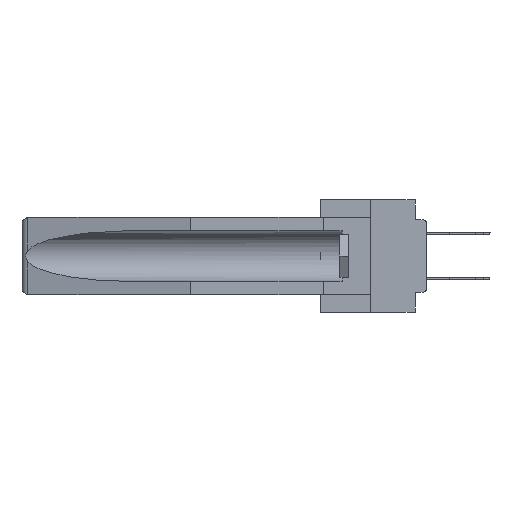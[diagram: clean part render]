
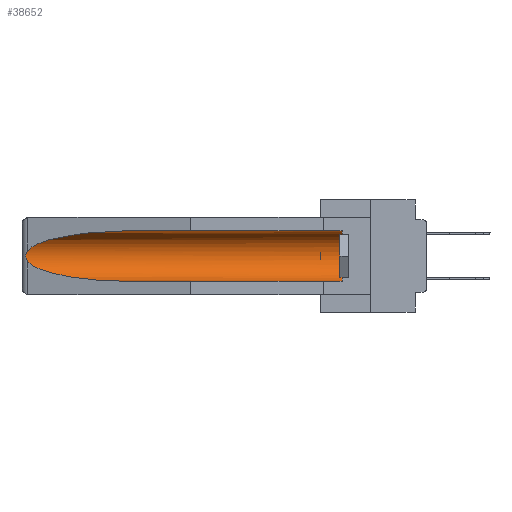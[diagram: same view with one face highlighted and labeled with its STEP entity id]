
A CAD part, left-side view. The second image highlights one B-rep face of the part: STEP entity #38652.
In plain terms, the highlighted cylindrical face has radius 2.857 mm (diameter 5.715 mm), a partial arc.
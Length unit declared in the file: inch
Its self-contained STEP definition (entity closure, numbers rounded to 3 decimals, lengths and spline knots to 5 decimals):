
#609 = CARTESIAN_POINT ( 'NONE',  ( 0.26654, 1.53092, -0.15636 ) ) ;
#806 = CARTESIAN_POINT ( 'NONE',  ( 0.26655, 1.53094, -0.18657 ) ) ;
#1081 = CARTESIAN_POINT ( 'NONE',  ( 0.26537, 1.52718, -0.14972 ) ) ;
#1139 = CARTESIAN_POINT ( 'NONE',  ( 0.155, -0.30754, -0.284 ) ) ;
#1728 = ORIENTED_EDGE ( 'NONE', *, *, #10005, .T. ) ;
#3050 = AXIS2_PLACEMENT_3D ( 'NONE', #12891, #9773, #9546 ) ;
#3756 = CARTESIAN_POINT ( 'NONE',  ( 0.26537, 1.52718, -0.14972 ) ) ;
#4275 = DIRECTION ( 'NONE',  ( 0., 1., 0. ) ) ;
#4434 = CARTESIAN_POINT ( 'NONE',  ( 0.155, 1.07973, -0.059 ) ) ;
#4891 = CARTESIAN_POINT ( 'NONE',  ( 0.155, -0.30754, -0.1715 ) ) ;
#5261 = CARTESIAN_POINT ( 'NONE',  ( 0.21114, 1.30732, -0.284 ) ) ;
#5456 = CARTESIAN_POINT ( 'NONE',  ( 0.26537, 1.52718, -0.19328 ) ) ;
#5550 = EDGE_CURVE ( 'NONE', #35433, #32252, #39615, .T. ) ;
#5663 = CARTESIAN_POINT ( 'NONE',  ( 0.155, 0.126, -0.284 ) ) ;
#6331 = EDGE_CURVE ( 'NONE', #32613, #35433, #33006, .T. ) ;
#7255 = VECTOR ( 'NONE', #4275, 39.37008 ) ;
#7978 = CARTESIAN_POINT ( 'NONE',  ( 0.155, 1.07973, -0.284 ) ) ;
#8008 = CARTESIAN_POINT ( 'NONE',  ( 0.155, 1.07973, -0.059 ) ) ;
#8222 = FACE_OUTER_BOUND ( 'NONE', #16572, .T. ) ;
#8805 = ORIENTED_EDGE ( 'NONE', *, *, #15074, .T. ) ;
#9546 = DIRECTION ( 'NONE',  ( 0., 0., 1. ) ) ;
#9773 = DIRECTION ( 'NONE',  ( 0., -1., 0. ) ) ;
#9837 = AXIS2_PLACEMENT_3D ( 'NONE', #4891, #21392, #27253 ) ;
#10005 = EDGE_CURVE ( 'NONE', #35949, #32613, #24362, .T. ) ;
#12891 = CARTESIAN_POINT ( 'NONE',  ( 0.155, 0.126, -0.1715 ) ) ;
#13347 = CARTESIAN_POINT ( 'NONE',  ( 0.2675, 1.53308, -0.17534 ) ) ;
#13971 = CARTESIAN_POINT ( 'NONE',  ( 0.155, 1.07973, -0.284 ) ) ;
#14422 = ORIENTED_EDGE ( 'NONE', *, *, #19055, .T. ) ;
#14538 = CARTESIAN_POINT ( 'NONE',  ( 0.2673, 1.53269, -0.17917 ) ) ;
#15074 = EDGE_CURVE ( 'NONE', #34534, #35949, #24434, .T. ) ;
#16488 = CARTESIAN_POINT ( 'NONE',  ( 0.26537, 1.52718, -0.19328 ) ) ;
#16572 = EDGE_LOOP ( 'NONE', ( #29019, #29913, #14422, #40373, #8805, #1728 ) ) ;
#16731 = CARTESIAN_POINT ( 'NONE',  ( 0.21114, 1.30732, -0.059 ) ) ;
#19055 = EDGE_CURVE ( 'NONE', #32252, #34837, #34350, .T. ) ;
#20766 = CYLINDRICAL_SURFACE ( 'NONE', #9837, 0.1125 ) ;
#20803 = CARTESIAN_POINT ( 'NONE',  ( 0.26597, 1.52961, -0.15275 ) ) ;
#21392 = DIRECTION ( 'NONE',  ( 0., 1., 0. ) ) ;
#24362 = LINE ( 'NONE', #38758, #38002 ) ;
#24382 = CARTESIAN_POINT ( 'NONE',  ( 0.26597, 1.5296, -0.19026 ) ) ;
#24434 = CIRCLE ( 'NONE', #3050, 0.1125 ) ;
#24600 = CARTESIAN_POINT ( 'NONE',  ( 0.26537, 1.52718, -0.14972 ) ) ;
#26148 = CARTESIAN_POINT ( 'NONE',  ( 0.155, 0.126, -0.059 ) ) ;
#27253 = DIRECTION ( 'NONE',  ( 0., 0., 1. ) ) ;
#29019 = ORIENTED_EDGE ( 'NONE', *, *, #6331, .T. ) ;
#29123 = DIRECTION ( 'NONE',  ( 0., 1., 0. ) ) ;
#29704 = CARTESIAN_POINT ( 'NONE',  ( 0.25451, 1.48313, -0.09465 ) ) ;
#29913 = ORIENTED_EDGE ( 'NONE', *, *, #5550, .T. ) ;
#32252 = VERTEX_POINT ( 'NONE', #33607 ) ;
#32613 = VERTEX_POINT ( 'NONE', #8008 ) ;
#33006 =( BOUNDED_CURVE ( )  B_SPLINE_CURVE ( 3, ( #4434, #16731, #29704, #1081 ),
 .UNSPECIFIED., .F., .T. ) 
 B_SPLINE_CURVE_WITH_KNOTS ( ( 4, 4 ),
 ( 4.71239, 6.08839 ),
 .UNSPECIFIED. ) 
 CURVE ( )  GEOMETRIC_REPRESENTATION_ITEM ( )  RATIONAL_B_SPLINE_CURVE ( ( 1., 0.848, 0.848, 1. ) ) 
 REPRESENTATION_ITEM ( '' )  );
#33556 = CARTESIAN_POINT ( 'NONE',  ( 0.2673, 1.5327, -0.16383 ) ) ;
#33607 = CARTESIAN_POINT ( 'NONE',  ( 0.26537, 1.52718, -0.19328 ) ) ;
#34350 =( BOUNDED_CURVE ( )  B_SPLINE_CURVE ( 3, ( #5456, #39998, #5261, #7978 ),
 .UNSPECIFIED., .F., .T. ) 
 B_SPLINE_CURVE_WITH_KNOTS ( ( 4, 4 ),
 ( 0.1948, 1.5708 ),
 .UNSPECIFIED. ) 
 CURVE ( )  GEOMETRIC_REPRESENTATION_ITEM ( )  RATIONAL_B_SPLINE_CURVE ( ( 1., 0.848, 0.848, 1. ) ) 
 REPRESENTATION_ITEM ( '' )  );
#34534 = VERTEX_POINT ( 'NONE', #5663 ) ;
#34837 = VERTEX_POINT ( 'NONE', #13971 ) ;
#35433 = VERTEX_POINT ( 'NONE', #24600 ) ;
#35599 = EDGE_CURVE ( 'NONE', #34534, #34837, #41324, .T. ) ;
#35949 = VERTEX_POINT ( 'NONE', #26148 ) ;
#38002 = VECTOR ( 'NONE', #29123, 39.37008 ) ;
#38652 = ADVANCED_FACE ( 'NONE', ( #8222 ), #20766, .F. ) ;
#38758 = CARTESIAN_POINT ( 'NONE',  ( 0.155, -0.30754, -0.059 ) ) ;
#38884 = CARTESIAN_POINT ( 'NONE',  ( 0.2675, 1.53308, -0.16763 ) ) ;
#39615 = B_SPLINE_CURVE_WITH_KNOTS ( 'NONE', 3,
 ( #3756, #20803, #609, #33556, #38884, #13347, #14538, #806, #24382, #16488 ),
 .UNSPECIFIED., .F., .F.,
 ( 4, 2, 2, 2, 4 ),
 ( 0., 0.00029, 0.00058, 0.00087, 0.00117 ),
 .UNSPECIFIED. ) ;
#39998 = CARTESIAN_POINT ( 'NONE',  ( 0.25451, 1.48313, -0.24835 ) ) ;
#40373 = ORIENTED_EDGE ( 'NONE', *, *, #35599, .F. ) ;
#41324 = LINE ( 'NONE', #1139, #7255 ) ;
